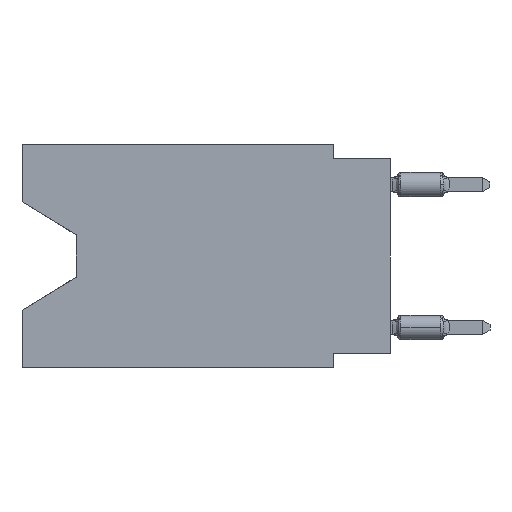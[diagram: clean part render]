
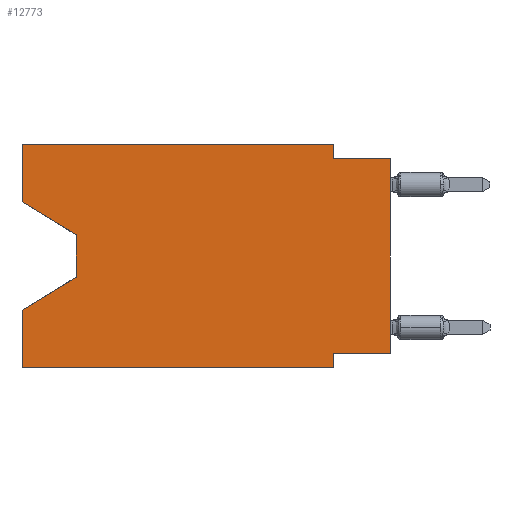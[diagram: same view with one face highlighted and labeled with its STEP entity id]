
A CAD part, left-side view. The second image highlights one B-rep face of the part: STEP entity #12773.
In plain terms, the highlighted planar face has unit normal (-1, 0, 0).
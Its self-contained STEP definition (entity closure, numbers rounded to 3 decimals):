
#17 = FACE_OUTER_BOUND ( 'NONE', #3849, .T. ) ;
#129 = VERTEX_POINT ( 'NONE', #13417 ) ;
#723 = DIRECTION ( 'NONE',  ( 0., -1., 0. ) ) ;
#894 = VECTOR ( 'NONE', #3478, 1000. ) ;
#960 = CARTESIAN_POINT ( 'NONE',  ( 0., 16.383, -9.906 ) ) ;
#1308 = CARTESIAN_POINT ( 'NONE',  ( 0., 0., -9.271 ) ) ;
#1488 = VECTOR ( 'NONE', #723, 1000. ) ;
#1495 = ORIENTED_EDGE ( 'NONE', *, *, #17223, .F. ) ;
#1973 = DIRECTION ( 'NONE',  ( 0., -0.855, -0.519 ) ) ;
#2317 = VECTOR ( 'NONE', #15735, 1000. ) ;
#2543 = CARTESIAN_POINT ( 'NONE',  ( 0., 13.97, -4.013 ) ) ;
#2970 = VERTEX_POINT ( 'NONE', #12881 ) ;
#3281 = VECTOR ( 'NONE', #14773, 1000. ) ;
#3380 = CARTESIAN_POINT ( 'NONE',  ( 0., 16.383, 0. ) ) ;
#3478 = DIRECTION ( 'NONE',  ( 0., 0., 1. ) ) ;
#3849 = EDGE_LOOP ( 'NONE', ( #20346, #12584, #10901, #11399, #9767, #7054, #1495, #15596, #12904, #20867, #9095, #10586 ) ) ;
#3906 = EDGE_CURVE ( 'NONE', #18004, #17973, #8749, .T. ) ;
#4302 = CARTESIAN_POINT ( 'NONE',  ( 0., 16.383, 0. ) ) ;
#4795 = CARTESIAN_POINT ( 'NONE',  ( 0., 16.383, 0. ) ) ;
#5060 = VECTOR ( 'NONE', #1973, 1000. ) ;
#5287 = VECTOR ( 'NONE', #12434, 1000. ) ;
#5935 = LINE ( 'NONE', #6049, #5060 ) ;
#6049 = CARTESIAN_POINT ( 'NONE',  ( 0., 16.383, -2.546 ) ) ;
#6618 = DIRECTION ( 'NONE',  ( 1., 0., 0. ) ) ;
#6648 = CARTESIAN_POINT ( 'NONE',  ( 0., 0., -9.271 ) ) ;
#6692 = VECTOR ( 'NONE', #17213, 1000. ) ;
#7054 = ORIENTED_EDGE ( 'NONE', *, *, #9060, .F. ) ;
#7649 = LINE ( 'NONE', #960, #6692 ) ;
#8139 = CARTESIAN_POINT ( 'NONE',  ( 0., 2.54, 0. ) ) ;
#8749 = LINE ( 'NONE', #20120, #21125 ) ;
#9044 = EDGE_CURVE ( 'NONE', #12920, #17973, #13556, .T. ) ;
#9060 = EDGE_CURVE ( 'NONE', #21026, #11738, #9877, .T. ) ;
#9095 = ORIENTED_EDGE ( 'NONE', *, *, #16628, .F. ) ;
#9515 = LINE ( 'NONE', #1308, #15059 ) ;
#9767 = ORIENTED_EDGE ( 'NONE', *, *, #13166, .T. ) ;
#9877 = LINE ( 'NONE', #18120, #14391 ) ;
#10505 = LINE ( 'NONE', #15939, #2317 ) ;
#10586 = ORIENTED_EDGE ( 'NONE', *, *, #12129, .F. ) ;
#10857 = AXIS2_PLACEMENT_3D ( 'NONE', #4795, #6618, #19318 ) ;
#10901 = ORIENTED_EDGE ( 'NONE', *, *, #3906, .T. ) ;
#11193 = PLANE ( 'NONE',  #10857 ) ;
#11248 = VECTOR ( 'NONE', #18645, 1000. ) ;
#11399 = ORIENTED_EDGE ( 'NONE', *, *, #9044, .F. ) ;
#11475 = EDGE_CURVE ( 'NONE', #2970, #17292, #21243, .T. ) ;
#11682 = LINE ( 'NONE', #18286, #12182 ) ;
#11706 = EDGE_CURVE ( 'NONE', #16966, #18004, #17241, .T. ) ;
#11738 = VERTEX_POINT ( 'NONE', #18855 ) ;
#11916 = DIRECTION ( 'NONE',  ( 0., 0.855, -0.519 ) ) ;
#12129 = EDGE_CURVE ( 'NONE', #129, #16829, #14167, .T. ) ;
#12150 = CARTESIAN_POINT ( 'NONE',  ( 0., 16.383, -9.906 ) ) ;
#12182 = VECTOR ( 'NONE', #17978, 1000. ) ;
#12434 = DIRECTION ( 'NONE',  ( 0., 0., 1. ) ) ;
#12584 = ORIENTED_EDGE ( 'NONE', *, *, #11706, .T. ) ;
#12773 = ADVANCED_FACE ( 'NONE', ( #17 ), #11193, .F. ) ;
#12881 = CARTESIAN_POINT ( 'NONE',  ( 0., 2.54, 0. ) ) ;
#12904 = ORIENTED_EDGE ( 'NONE', *, *, #14242, .F. ) ;
#12920 = VERTEX_POINT ( 'NONE', #12150 ) ;
#13166 = EDGE_CURVE ( 'NONE', #12920, #11738, #7649, .T. ) ;
#13417 = CARTESIAN_POINT ( 'NONE',  ( 0., 16.383, -2.546 ) ) ;
#13556 = LINE ( 'NONE', #3380, #894 ) ;
#14167 = LINE ( 'NONE', #4302, #5287 ) ;
#14242 = EDGE_CURVE ( 'NONE', #17292, #18126, #11682, .T. ) ;
#14391 = VECTOR ( 'NONE', #14774, 1000. ) ;
#14586 = CARTESIAN_POINT ( 'NONE',  ( 0., 2.54, -9.271 ) ) ;
#14773 = DIRECTION ( 'NONE',  ( 0., 0., -1. ) ) ;
#14774 = DIRECTION ( 'NONE',  ( 0., 0., -1. ) ) ;
#14993 = CARTESIAN_POINT ( 'NONE',  ( 0., 2.54, -0.635 ) ) ;
#15059 = VECTOR ( 'NONE', #17884, 1000. ) ;
#15262 = LINE ( 'NONE', #18819, #1488 ) ;
#15596 = ORIENTED_EDGE ( 'NONE', *, *, #18185, .T. ) ;
#15735 = DIRECTION ( 'NONE',  ( 0., 0., 1. ) ) ;
#15816 = CARTESIAN_POINT ( 'NONE',  ( 0., 16.383, 0. ) ) ;
#15891 = CARTESIAN_POINT ( 'NONE',  ( 0., 13.97, -5.893 ) ) ;
#15939 = CARTESIAN_POINT ( 'NONE',  ( 0., 0., 0. ) ) ;
#16487 = CARTESIAN_POINT ( 'NONE',  ( 0., 16.383, -7.36 ) ) ;
#16628 = EDGE_CURVE ( 'NONE', #16829, #2970, #15262, .T. ) ;
#16690 = CARTESIAN_POINT ( 'NONE',  ( 0., 0., -0.635 ) ) ;
#16829 = VERTEX_POINT ( 'NONE', #15816 ) ;
#16966 = VERTEX_POINT ( 'NONE', #2543 ) ;
#17213 = DIRECTION ( 'NONE',  ( 0., -1., 0. ) ) ;
#17223 = EDGE_CURVE ( 'NONE', #21217, #21026, #9515, .T. ) ;
#17241 = LINE ( 'NONE', #20464, #11248 ) ;
#17292 = VERTEX_POINT ( 'NONE', #14993 ) ;
#17884 = DIRECTION ( 'NONE',  ( 0., 1., 0. ) ) ;
#17973 = VERTEX_POINT ( 'NONE', #16487 ) ;
#17978 = DIRECTION ( 'NONE',  ( 0., -1., 0. ) ) ;
#18004 = VERTEX_POINT ( 'NONE', #15891 ) ;
#18120 = CARTESIAN_POINT ( 'NONE',  ( 0., 2.54, -9.906 ) ) ;
#18126 = VERTEX_POINT ( 'NONE', #16690 ) ;
#18185 = EDGE_CURVE ( 'NONE', #21217, #18126, #10505, .T. ) ;
#18286 = CARTESIAN_POINT ( 'NONE',  ( 0., 0., -0.635 ) ) ;
#18645 = DIRECTION ( 'NONE',  ( 0., 0., -1. ) ) ;
#18819 = CARTESIAN_POINT ( 'NONE',  ( 0., 16.383, 0. ) ) ;
#18855 = CARTESIAN_POINT ( 'NONE',  ( 0., 2.54, -9.906 ) ) ;
#19318 = DIRECTION ( 'NONE',  ( 0., 0., -1. ) ) ;
#19799 = EDGE_CURVE ( 'NONE', #129, #16966, #5935, .T. ) ;
#20120 = CARTESIAN_POINT ( 'NONE',  ( 0., 13.97, -5.893 ) ) ;
#20346 = ORIENTED_EDGE ( 'NONE', *, *, #19799, .T. ) ;
#20464 = CARTESIAN_POINT ( 'NONE',  ( 0., 13.97, -4.013 ) ) ;
#20867 = ORIENTED_EDGE ( 'NONE', *, *, #11475, .F. ) ;
#21026 = VERTEX_POINT ( 'NONE', #14586 ) ;
#21125 = VECTOR ( 'NONE', #11916, 1000. ) ;
#21217 = VERTEX_POINT ( 'NONE', #6648 ) ;
#21243 = LINE ( 'NONE', #8139, #3281 ) ;
